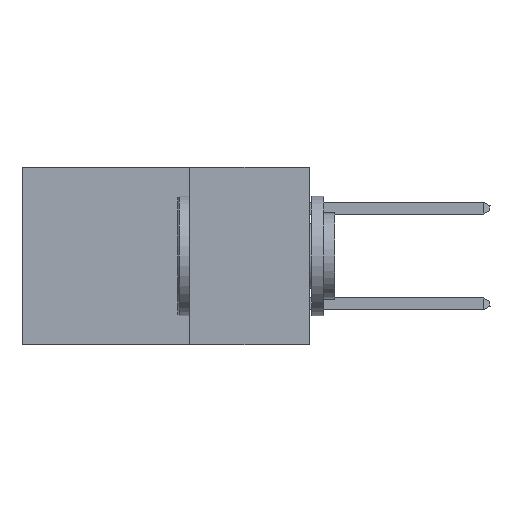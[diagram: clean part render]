
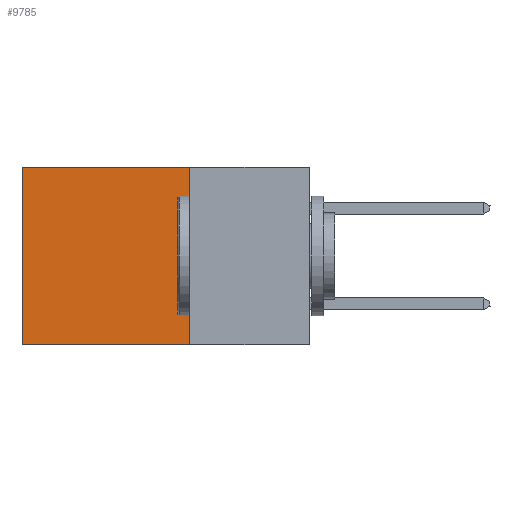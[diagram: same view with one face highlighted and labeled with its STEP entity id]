
A CAD part, left-side view. The second image highlights one B-rep face of the part: STEP entity #9785.
In plain terms, the highlighted planar face has unit normal (-1, 0, 0).
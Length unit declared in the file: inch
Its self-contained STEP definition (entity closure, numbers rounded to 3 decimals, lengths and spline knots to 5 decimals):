
#18 = VECTOR ( 'NONE', #490, 39.37008 ) ;
#139 = VERTEX_POINT ( 'NONE', #4756 ) ;
#374 = CARTESIAN_POINT ( 'NONE',  ( 0.2875, 0.25, 0. ) ) ;
#490 = DIRECTION ( 'NONE',  ( 0., 1., 0. ) ) ;
#514 = VECTOR ( 'NONE', #8715, 39.37008 ) ;
#552 = AXIS2_PLACEMENT_3D ( 'NONE', #374, #1381, #7925 ) ;
#884 = CARTESIAN_POINT ( 'NONE',  ( 0.2875, 0.25, -0.37 ) ) ;
#1381 = DIRECTION ( 'NONE',  ( 1., 0., 0. ) ) ;
#2036 = VECTOR ( 'NONE', #7450, 39.37008 ) ;
#2051 = VERTEX_POINT ( 'NONE', #6115 ) ;
#2347 = LINE ( 'NONE', #6136, #18 ) ;
#2853 = VERTEX_POINT ( 'NONE', #7877 ) ;
#3122 = CARTESIAN_POINT ( 'NONE',  ( 0.2875, 0.6, 0. ) ) ;
#3394 = LINE ( 'NONE', #8873, #7774 ) ;
#4227 = DIRECTION ( 'NONE',  ( 0., 0., -1. ) ) ;
#4387 = FACE_OUTER_BOUND ( 'NONE', #11917, .T. ) ;
#4756 = CARTESIAN_POINT ( 'NONE',  ( 0.2875, 0.25, 0. ) ) ;
#5804 = EDGE_CURVE ( 'NONE', #139, #2051, #2347, .T. ) ;
#6041 = PLANE ( 'NONE',  #552 ) ;
#6115 = CARTESIAN_POINT ( 'NONE',  ( 0.2875, 0.6, 0. ) ) ;
#6136 = CARTESIAN_POINT ( 'NONE',  ( 0.2875, 0.25, 0. ) ) ;
#6703 = LINE ( 'NONE', #884, #2036 ) ;
#6792 = VERTEX_POINT ( 'NONE', #12165 ) ;
#7421 = EDGE_CURVE ( 'NONE', #2853, #6792, #6703, .T. ) ;
#7450 = DIRECTION ( 'NONE',  ( 0., 1., 0. ) ) ;
#7774 = VECTOR ( 'NONE', #4227, 39.37008 ) ;
#7877 = CARTESIAN_POINT ( 'NONE',  ( 0.2875, 0.25, -0.37 ) ) ;
#7925 = DIRECTION ( 'NONE',  ( 0., 0., -1. ) ) ;
#8214 = ORIENTED_EDGE ( 'NONE', *, *, #7421, .F. ) ;
#8325 = EDGE_CURVE ( 'NONE', #139, #2853, #3394, .T. ) ;
#8609 = ORIENTED_EDGE ( 'NONE', *, *, #9684, .T. ) ;
#8715 = DIRECTION ( 'NONE',  ( 0., 0., -1. ) ) ;
#8873 = CARTESIAN_POINT ( 'NONE',  ( 0.2875, 0.25, 0. ) ) ;
#9684 = EDGE_CURVE ( 'NONE', #2051, #6792, #10525, .T. ) ;
#9785 = ADVANCED_FACE ( 'NONE', ( #4387 ), #6041, .F. ) ;
#9869 = ORIENTED_EDGE ( 'NONE', *, *, #8325, .F. ) ;
#10525 = LINE ( 'NONE', #3122, #514 ) ;
#11755 = ORIENTED_EDGE ( 'NONE', *, *, #5804, .T. ) ;
#11917 = EDGE_LOOP ( 'NONE', ( #8609, #8214, #9869, #11755 ) ) ;
#12165 = CARTESIAN_POINT ( 'NONE',  ( 0.2875, 0.6, -0.37 ) ) ;
